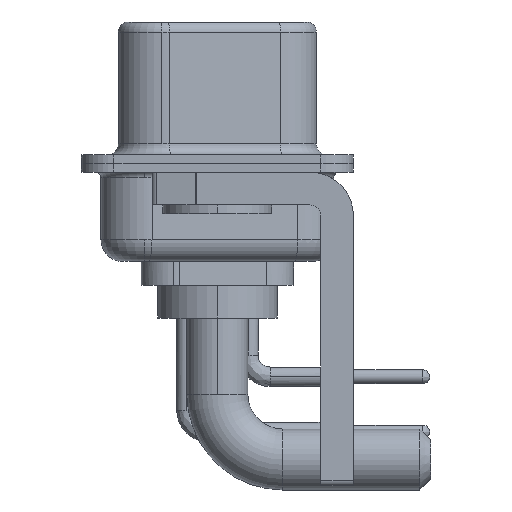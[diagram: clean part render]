
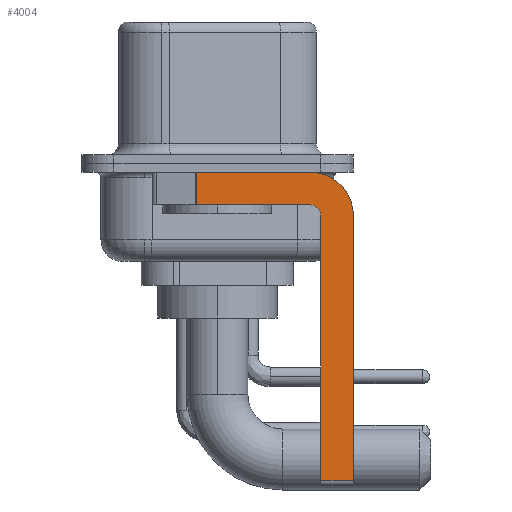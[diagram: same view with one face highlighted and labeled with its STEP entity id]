
A CAD part, left-side view. The second image highlights one B-rep face of the part: STEP entity #4004.
In plain terms, the highlighted planar face has unit normal (-1, 0, 0).
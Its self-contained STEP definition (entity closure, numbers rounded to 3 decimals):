
#62 = VECTOR ( 'NONE', #5809, 1000. ) ;
#122 = CARTESIAN_POINT ( 'NONE',  ( -2.9, -4.25, -1.9 ) ) ;
#138 = AXIS2_PLACEMENT_3D ( 'NONE', #14281, #2541, #12745 ) ;
#332 = DIRECTION ( 'NONE',  ( 0., 1., 0. ) ) ;
#1501 = VECTOR ( 'NONE', #16749, 1000. ) ;
#2541 = DIRECTION ( 'NONE',  ( 1., 0., 0. ) ) ;
#2680 = DIRECTION ( 'NONE',  ( 0., 0., -1. ) ) ;
#2903 = CARTESIAN_POINT ( 'NONE',  ( -2.9, -4.25, -2.4 ) ) ;
#3099 = CARTESIAN_POINT ( 'NONE',  ( -2.9, -4.25, -0.4 ) ) ;
#3369 = CARTESIAN_POINT ( 'NONE',  ( -2.9, 0.978, -1.9 ) ) ;
#4004 = ADVANCED_FACE ( 'NONE', ( #19358 ), #17821, .F. ) ;
#5249 = CARTESIAN_POINT ( 'NONE',  ( -2.9, -4.75, -14.55 ) ) ;
#5603 = DIRECTION ( 'NONE',  ( -1., 0., 0. ) ) ;
#5766 = LINE ( 'NONE', #16180, #21133 ) ;
#5809 = DIRECTION ( 'NONE',  ( 0., -1., 0. ) ) ;
#6698 = LINE ( 'NONE', #15482, #9430 ) ;
#6788 = AXIS2_PLACEMENT_3D ( 'NONE', #10443, #5603, #9000 ) ;
#6892 = EDGE_CURVE ( 'NONE', #8790, #10383, #18357, .T. ) ;
#6968 = EDGE_CURVE ( 'NONE', #15876, #15213, #14870, .T. ) ;
#7689 = LINE ( 'NONE', #12659, #12097 ) ;
#7706 = DIRECTION ( 'NONE',  ( 0., 0., 1. ) ) ;
#8496 = AXIS2_PLACEMENT_3D ( 'NONE', #2903, #20903, #2680 ) ;
#8533 = ORIENTED_EDGE ( 'NONE', *, *, #6892, .F. ) ;
#8790 = VERTEX_POINT ( 'NONE', #14160 ) ;
#8856 = CARTESIAN_POINT ( 'NONE',  ( -2.9, -6.25, -2.4 ) ) ;
#9000 = DIRECTION ( 'NONE',  ( 0., 0., 1. ) ) ;
#9430 = VECTOR ( 'NONE', #332, 1000. ) ;
#10060 = CARTESIAN_POINT ( 'NONE',  ( -2.9, -6.25, -14.55 ) ) ;
#10383 = VERTEX_POINT ( 'NONE', #122 ) ;
#10394 = EDGE_CURVE ( 'NONE', #10383, #19025, #6698, .T. ) ;
#10443 = CARTESIAN_POINT ( 'NONE',  ( -2.9, -4.25, -2.4 ) ) ;
#10790 = ORIENTED_EDGE ( 'NONE', *, *, #17745, .T. ) ;
#12097 = VECTOR ( 'NONE', #19239, 1000. ) ;
#12297 = LINE ( 'NONE', #20953, #62 ) ;
#12436 = VECTOR ( 'NONE', #18172, 1000. ) ;
#12659 = CARTESIAN_POINT ( 'NONE',  ( -2.9, 3., -0.4 ) ) ;
#12745 = DIRECTION ( 'NONE',  ( 0., 0., -1. ) ) ;
#13246 = LINE ( 'NONE', #3369, #1501 ) ;
#13472 = CARTESIAN_POINT ( 'NONE',  ( -2.9, -6.25, -2.4 ) ) ;
#14160 = CARTESIAN_POINT ( 'NONE',  ( -2.9, -4.75, -2.4 ) ) ;
#14242 = EDGE_LOOP ( 'NONE', ( #15009, #14592, #18391, #8533, #18460, #10790, #18272, #20139 ) ) ;
#14281 = CARTESIAN_POINT ( 'NONE',  ( -2.9, -4.25, -2.4 ) ) ;
#14423 = VERTEX_POINT ( 'NONE', #20980 ) ;
#14592 = ORIENTED_EDGE ( 'NONE', *, *, #18514, .T. ) ;
#14870 = CIRCLE ( 'NONE', #138, 2. ) ;
#14894 = LINE ( 'NONE', #13472, #12436 ) ;
#15009 = ORIENTED_EDGE ( 'NONE', *, *, #20382, .F. ) ;
#15213 = VERTEX_POINT ( 'NONE', #8856 ) ;
#15482 = CARTESIAN_POINT ( 'NONE',  ( -2.9, -4.25, -1.9 ) ) ;
#15876 = VERTEX_POINT ( 'NONE', #3099 ) ;
#16180 = CARTESIAN_POINT ( 'NONE',  ( -2.9, -4.75, -14.8 ) ) ;
#16749 = DIRECTION ( 'NONE',  ( 0., 0., -1. ) ) ;
#16820 = EDGE_CURVE ( 'NONE', #21229, #8790, #5766, .T. ) ;
#17745 = EDGE_CURVE ( 'NONE', #21229, #21638, #12297, .T. ) ;
#17821 = PLANE ( 'NONE',  #8496 ) ;
#18172 = DIRECTION ( 'NONE',  ( 0., 0., -1. ) ) ;
#18272 = ORIENTED_EDGE ( 'NONE', *, *, #19766, .F. ) ;
#18357 = CIRCLE ( 'NONE', #6788, 0.5 ) ;
#18391 = ORIENTED_EDGE ( 'NONE', *, *, #10394, .F. ) ;
#18460 = ORIENTED_EDGE ( 'NONE', *, *, #16820, .F. ) ;
#18514 = EDGE_CURVE ( 'NONE', #14423, #19025, #13246, .T. ) ;
#19025 = VERTEX_POINT ( 'NONE', #21179 ) ;
#19239 = DIRECTION ( 'NONE',  ( 0., -1., 0. ) ) ;
#19358 = FACE_OUTER_BOUND ( 'NONE', #14242, .T. ) ;
#19766 = EDGE_CURVE ( 'NONE', #15213, #21638, #14894, .T. ) ;
#20139 = ORIENTED_EDGE ( 'NONE', *, *, #6968, .F. ) ;
#20382 = EDGE_CURVE ( 'NONE', #14423, #15876, #7689, .T. ) ;
#20903 = DIRECTION ( 'NONE',  ( 1., 0., 0. ) ) ;
#20953 = CARTESIAN_POINT ( 'NONE',  ( -2.9, -4.25, -14.55 ) ) ;
#20980 = CARTESIAN_POINT ( 'NONE',  ( -2.9, 0.978, -0.4 ) ) ;
#21133 = VECTOR ( 'NONE', #7706, 1000. ) ;
#21179 = CARTESIAN_POINT ( 'NONE',  ( -2.9, 0.978, -1.9 ) ) ;
#21229 = VERTEX_POINT ( 'NONE', #5249 ) ;
#21638 = VERTEX_POINT ( 'NONE', #10060 ) ;
